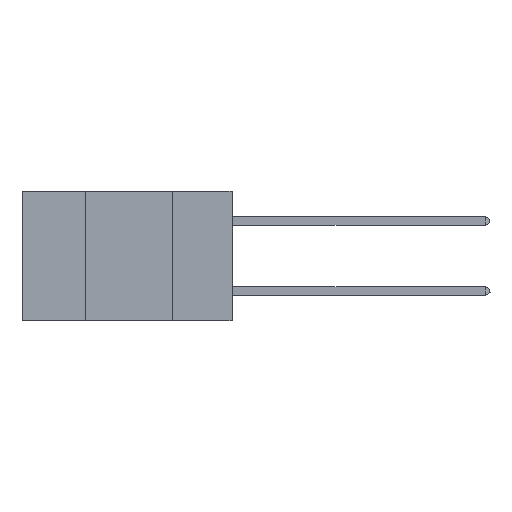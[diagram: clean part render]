
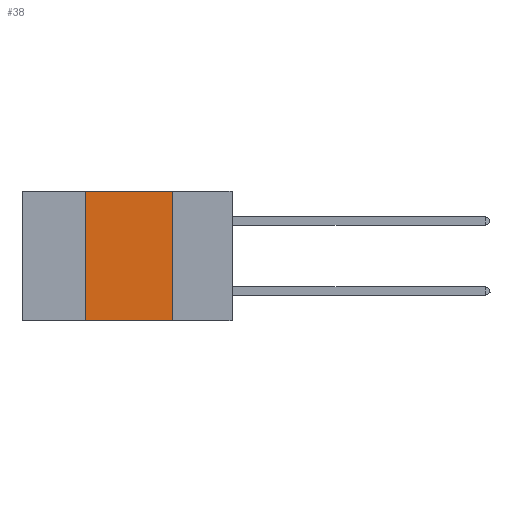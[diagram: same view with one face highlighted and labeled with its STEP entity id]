
A CAD part, left-side view. The second image highlights one B-rep face of the part: STEP entity #38.
In plain terms, the highlighted planar face has unit normal (-1, 0, 0).
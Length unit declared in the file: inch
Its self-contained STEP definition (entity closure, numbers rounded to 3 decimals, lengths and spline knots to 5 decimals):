
#38 = ADVANCED_FACE ( 'NONE', ( #11164 ), #1022, .F. ) ;
#63 = VERTEX_POINT ( 'NONE', #8171 ) ;
#517 = LINE ( 'NONE', #8239, #12144 ) ;
#736 = DIRECTION ( 'NONE',  ( 0., -1., 0. ) ) ;
#814 = CARTESIAN_POINT ( 'NONE',  ( 0., 0.42, 0. ) ) ;
#1022 = PLANE ( 'NONE',  #8218 ) ;
#1042 = LINE ( 'NONE', #9693, #2492 ) ;
#1190 = ORIENTED_EDGE ( 'NONE', *, *, #12649, .F. ) ;
#2204 = DIRECTION ( 'NONE',  ( 0., 0., -1. ) ) ;
#2492 = VECTOR ( 'NONE', #13110, 39.37008 ) ;
#4207 = EDGE_CURVE ( 'NONE', #63, #12795, #12728, .T. ) ;
#4874 = ORIENTED_EDGE ( 'NONE', *, *, #5716, .F. ) ;
#5716 = EDGE_CURVE ( 'NONE', #6860, #8591, #517, .T. ) ;
#6462 = EDGE_CURVE ( 'NONE', #8591, #12795, #8401, .T. ) ;
#6542 = CARTESIAN_POINT ( 'NONE',  ( 0., 0.6, -0.37 ) ) ;
#6860 = VERTEX_POINT ( 'NONE', #814 ) ;
#7578 = CARTESIAN_POINT ( 'NONE',  ( 0., 0.17, -0.37 ) ) ;
#8171 = CARTESIAN_POINT ( 'NONE',  ( 0., 0.42, -0.37 ) ) ;
#8218 = AXIS2_PLACEMENT_3D ( 'NONE', #12417, #8936, #11233 ) ;
#8239 = CARTESIAN_POINT ( 'NONE',  ( 0., 0.6, 0. ) ) ;
#8401 = LINE ( 'NONE', #11299, #12121 ) ;
#8591 = VERTEX_POINT ( 'NONE', #11339 ) ;
#8936 = DIRECTION ( 'NONE',  ( 1., 0., 0. ) ) ;
#9232 = VECTOR ( 'NONE', #14203, 39.37008 ) ;
#9693 = CARTESIAN_POINT ( 'NONE',  ( 0., 0.42, 0. ) ) ;
#11164 = FACE_OUTER_BOUND ( 'NONE', #13869, .T. ) ;
#11233 = DIRECTION ( 'NONE',  ( 0., 0., -1. ) ) ;
#11299 = CARTESIAN_POINT ( 'NONE',  ( 0., 0.17, 0. ) ) ;
#11339 = CARTESIAN_POINT ( 'NONE',  ( 0., 0.17, 0. ) ) ;
#12121 = VECTOR ( 'NONE', #2204, 39.37008 ) ;
#12144 = VECTOR ( 'NONE', #736, 39.37008 ) ;
#12417 = CARTESIAN_POINT ( 'NONE',  ( 0., 0.6, 0. ) ) ;
#12649 = EDGE_CURVE ( 'NONE', #63, #6860, #1042, .T. ) ;
#12728 = LINE ( 'NONE', #6542, #9232 ) ;
#12795 = VERTEX_POINT ( 'NONE', #7578 ) ;
#13110 = DIRECTION ( 'NONE',  ( 0., 0., 1. ) ) ;
#13869 = EDGE_LOOP ( 'NONE', ( #14339, #4874, #1190, #14024 ) ) ;
#14024 = ORIENTED_EDGE ( 'NONE', *, *, #4207, .T. ) ;
#14203 = DIRECTION ( 'NONE',  ( 0., -1., 0. ) ) ;
#14339 = ORIENTED_EDGE ( 'NONE', *, *, #6462, .F. ) ;
